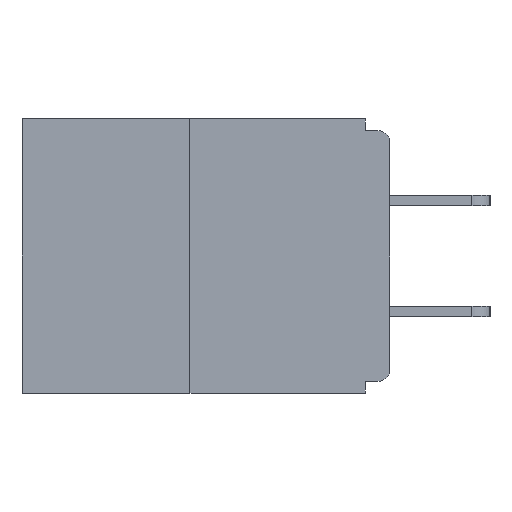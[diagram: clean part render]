
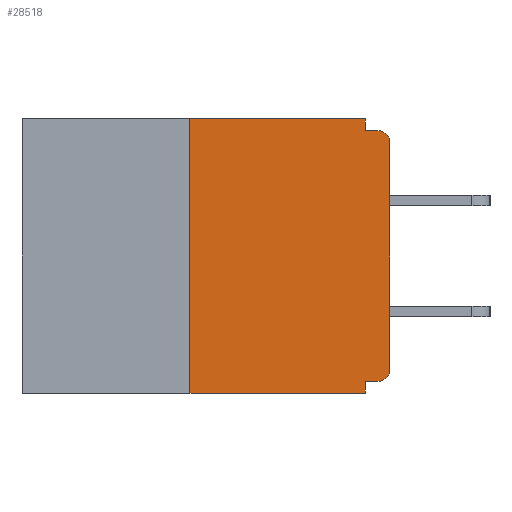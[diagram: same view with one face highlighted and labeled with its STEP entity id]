
A CAD part, left-side view. The second image highlights one B-rep face of the part: STEP entity #28518.
In plain terms, the highlighted planar face has unit normal (-1, 0, 0).
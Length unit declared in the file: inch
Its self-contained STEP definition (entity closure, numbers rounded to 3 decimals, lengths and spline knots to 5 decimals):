
#1296 = LINE ( 'NONE', #13578, #10542 ) ;
#2380 = CARTESIAN_POINT ( 'NONE',  ( 0., 0.031, 0. ) ) ;
#2612 = EDGE_CURVE ( 'NONE', #9870, #13940, #18368, .T. ) ;
#2633 = ORIENTED_EDGE ( 'NONE', *, *, #5515, .T. ) ;
#2938 = ORIENTED_EDGE ( 'NONE', *, *, #12225, .T. ) ;
#3331 = CARTESIAN_POINT ( 'NONE',  ( 0., 0.015, -0.328 ) ) ;
#3415 = PLANE ( 'NONE',  #21949 ) ;
#3678 = CIRCLE ( 'NONE', #12487, 0.015 ) ;
#4004 = CARTESIAN_POINT ( 'NONE',  ( 0., 0.46, 0. ) ) ;
#4087 = DIRECTION ( 'NONE',  ( 0., -1., 0. ) ) ;
#4602 = EDGE_CURVE ( 'NONE', #11225, #16689, #3678, .T. ) ;
#5407 = EDGE_LOOP ( 'NONE', ( #8462, #10579, #27047, #7941, #29664, #7583, #2938, #2633, #17812, #21696 ) ) ;
#5515 = EDGE_CURVE ( 'NONE', #22927, #12919, #19406, .T. ) ;
#6024 = VERTEX_POINT ( 'NONE', #17650 ) ;
#6059 = AXIS2_PLACEMENT_3D ( 'NONE', #7839, #12907, #17080 ) ;
#6194 = EDGE_CURVE ( 'NONE', #22091, #10007, #23770, .T. ) ;
#6201 = VECTOR ( 'NONE', #12456, 39.37008 ) ;
#6500 = CARTESIAN_POINT ( 'NONE',  ( 0., 0., -0.03 ) ) ;
#6507 = EDGE_CURVE ( 'NONE', #22091, #9870, #1296, .T. ) ;
#7529 = CARTESIAN_POINT ( 'NONE',  ( 0., 0.031, 0. ) ) ;
#7583 = ORIENTED_EDGE ( 'NONE', *, *, #4602, .T. ) ;
#7839 = CARTESIAN_POINT ( 'NONE',  ( 0., 0.015, -0.03 ) ) ;
#7941 = ORIENTED_EDGE ( 'NONE', *, *, #22906, .F. ) ;
#8462 = ORIENTED_EDGE ( 'NONE', *, *, #2612, .F. ) ;
#8803 = DIRECTION ( 'NONE',  ( 0., 0., -1. ) ) ;
#9524 = CARTESIAN_POINT ( 'NONE',  ( 0., 0.031, -0.343 ) ) ;
#9691 = DIRECTION ( 'NONE',  ( -1., 0., 0. ) ) ;
#9870 = VERTEX_POINT ( 'NONE', #29275 ) ;
#10007 = VERTEX_POINT ( 'NONE', #9524 ) ;
#10268 = CARTESIAN_POINT ( 'NONE',  ( 0., 0.015, -0.015 ) ) ;
#10542 = VECTOR ( 'NONE', #29762, 39.37008 ) ;
#10579 = ORIENTED_EDGE ( 'NONE', *, *, #6507, .F. ) ;
#10593 = DIRECTION ( 'NONE',  ( 1., 0., 0. ) ) ;
#11203 = DIRECTION ( 'NONE',  ( 0., -1., 0. ) ) ;
#11225 = VERTEX_POINT ( 'NONE', #3331 ) ;
#11398 = LINE ( 'NONE', #20321, #14204 ) ;
#11424 = CARTESIAN_POINT ( 'NONE',  ( 0., 0., 0. ) ) ;
#11561 = LINE ( 'NONE', #30359, #22446 ) ;
#12065 = CARTESIAN_POINT ( 'NONE',  ( 0., 0.46, -0.343 ) ) ;
#12225 = EDGE_CURVE ( 'NONE', #16689, #22927, #18343, .T. ) ;
#12456 = DIRECTION ( 'NONE',  ( 0., 0., -1. ) ) ;
#12487 = AXIS2_PLACEMENT_3D ( 'NONE', #21563, #9691, #28343 ) ;
#12907 = DIRECTION ( 'NONE',  ( -1., 0., 0. ) ) ;
#12919 = VERTEX_POINT ( 'NONE', #10268 ) ;
#13063 = VECTOR ( 'NONE', #23130, 39.37008 ) ;
#13354 = CARTESIAN_POINT ( 'NONE',  ( 0., 0., -0.015 ) ) ;
#13467 = VECTOR ( 'NONE', #19157, 39.37008 ) ;
#13578 = CARTESIAN_POINT ( 'NONE',  ( 0., 0.25, 0. ) ) ;
#13940 = VERTEX_POINT ( 'NONE', #2380 ) ;
#14204 = VECTOR ( 'NONE', #16011, 39.37008 ) ;
#14465 = LINE ( 'NONE', #7529, #6201 ) ;
#16011 = DIRECTION ( 'NONE',  ( 0., 1., 0. ) ) ;
#16689 = VERTEX_POINT ( 'NONE', #17621 ) ;
#17080 = DIRECTION ( 'NONE',  ( 0., 0., -1. ) ) ;
#17570 = VECTOR ( 'NONE', #4087, 39.37008 ) ;
#17621 = CARTESIAN_POINT ( 'NONE',  ( 0., 0., -0.313 ) ) ;
#17650 = CARTESIAN_POINT ( 'NONE',  ( 0., 0.031, -0.328 ) ) ;
#17812 = ORIENTED_EDGE ( 'NONE', *, *, #25955, .F. ) ;
#18343 = LINE ( 'NONE', #11424, #13063 ) ;
#18368 = LINE ( 'NONE', #25480, #17570 ) ;
#19157 = DIRECTION ( 'NONE',  ( 0., -1., 0. ) ) ;
#19406 = CIRCLE ( 'NONE', #6059, 0.015 ) ;
#20154 = FACE_OUTER_BOUND ( 'NONE', #5407, .T. ) ;
#20321 = CARTESIAN_POINT ( 'NONE',  ( 0., 0., -0.328 ) ) ;
#21043 = CARTESIAN_POINT ( 'NONE',  ( 0., 0.25, -0.343 ) ) ;
#21563 = CARTESIAN_POINT ( 'NONE',  ( 0., 0.015, -0.313 ) ) ;
#21696 = ORIENTED_EDGE ( 'NONE', *, *, #28312, .F. ) ;
#21949 = AXIS2_PLACEMENT_3D ( 'NONE', #4004, #10593, #24773 ) ;
#22091 = VERTEX_POINT ( 'NONE', #21043 ) ;
#22445 = LINE ( 'NONE', #13354, #29912 ) ;
#22446 = VECTOR ( 'NONE', #8803, 39.37008 ) ;
#22472 = VERTEX_POINT ( 'NONE', #27955 ) ;
#22906 = EDGE_CURVE ( 'NONE', #6024, #10007, #11561, .T. ) ;
#22927 = VERTEX_POINT ( 'NONE', #6500 ) ;
#23130 = DIRECTION ( 'NONE',  ( 0., 0., 1. ) ) ;
#23770 = LINE ( 'NONE', #12065, #13467 ) ;
#24773 = DIRECTION ( 'NONE',  ( 0., 0., -1. ) ) ;
#25480 = CARTESIAN_POINT ( 'NONE',  ( 0., 0.46, 0. ) ) ;
#25955 = EDGE_CURVE ( 'NONE', #22472, #12919, #22445, .T. ) ;
#26817 = EDGE_CURVE ( 'NONE', #11225, #6024, #11398, .T. ) ;
#27047 = ORIENTED_EDGE ( 'NONE', *, *, #6194, .T. ) ;
#27955 = CARTESIAN_POINT ( 'NONE',  ( 0., 0.031, -0.015 ) ) ;
#28312 = EDGE_CURVE ( 'NONE', #13940, #22472, #14465, .T. ) ;
#28343 = DIRECTION ( 'NONE',  ( 0., 0., -1. ) ) ;
#28518 = ADVANCED_FACE ( 'NONE', ( #20154 ), #3415, .F. ) ;
#29275 = CARTESIAN_POINT ( 'NONE',  ( 0., 0.25, 0. ) ) ;
#29664 = ORIENTED_EDGE ( 'NONE', *, *, #26817, .F. ) ;
#29762 = DIRECTION ( 'NONE',  ( 0., 0., 1. ) ) ;
#29912 = VECTOR ( 'NONE', #11203, 39.37008 ) ;
#30359 = CARTESIAN_POINT ( 'NONE',  ( 0., 0.031, -0.343 ) ) ;
